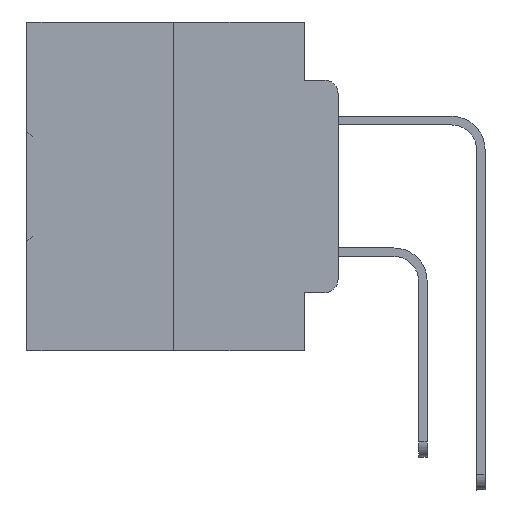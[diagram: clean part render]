
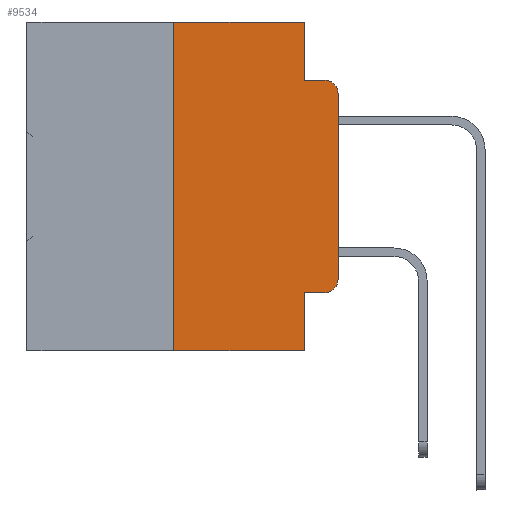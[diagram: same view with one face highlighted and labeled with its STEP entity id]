
A CAD part, left-side view. The second image highlights one B-rep face of the part: STEP entity #9534.
In plain terms, the highlighted planar face has unit normal (-1, 0, 0).
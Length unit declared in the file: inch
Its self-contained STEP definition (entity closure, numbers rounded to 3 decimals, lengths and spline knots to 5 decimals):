
#458 = CARTESIAN_POINT ( 'NONE',  ( 0., 0.25, -0.5 ) ) ;
#621 = ORIENTED_EDGE ( 'NONE', *, *, #17937, .F. ) ;
#1419 = VECTOR ( 'NONE', #21801, 39.37008 ) ;
#1692 = AXIS2_PLACEMENT_3D ( 'NONE', #29092, #12473, #31791 ) ;
#1959 = EDGE_CURVE ( 'NONE', #13216, #26898, #23651, .T. ) ;
#2672 = DIRECTION ( 'NONE',  ( 0., 0., -1. ) ) ;
#3133 = CARTESIAN_POINT ( 'NONE',  ( 0., 0.473, 0. ) ) ;
#4731 = DIRECTION ( 'NONE',  ( 0., -1., 0. ) ) ;
#5569 = ORIENTED_EDGE ( 'NONE', *, *, #9175, .T. ) ;
#5949 = CARTESIAN_POINT ( 'NONE',  ( 0., 0.02, -0.3915 ) ) ;
#6005 = DIRECTION ( 'NONE',  ( 0., -1., 0. ) ) ;
#6190 = ORIENTED_EDGE ( 'NONE', *, *, #30833, .T. ) ;
#6446 = CARTESIAN_POINT ( 'NONE',  ( 0., 0.473, -0.5 ) ) ;
#6785 = CARTESIAN_POINT ( 'NONE',  ( 0., 0.051, -0.4115 ) ) ;
#7320 = LINE ( 'NONE', #27417, #8239 ) ;
#7840 = VECTOR ( 'NONE', #34298, 39.37008 ) ;
#8078 = AXIS2_PLACEMENT_3D ( 'NONE', #5949, #25584, #8837 ) ;
#8204 = LINE ( 'NONE', #13092, #22275 ) ;
#8239 = VECTOR ( 'NONE', #10777, 39.37008 ) ;
#8837 = DIRECTION ( 'NONE',  ( 0., 0., -1. ) ) ;
#8982 = CARTESIAN_POINT ( 'NONE',  ( 0., 0., -0.3915 ) ) ;
#9175 = EDGE_CURVE ( 'NONE', #9709, #26898, #31690, .T. ) ;
#9199 = CARTESIAN_POINT ( 'NONE',  ( 0., 0., -0.1085 ) ) ;
#9534 = ADVANCED_FACE ( 'NONE', ( #34170 ), #14041, .F. ) ;
#9709 = VERTEX_POINT ( 'NONE', #9199 ) ;
#9839 = ORIENTED_EDGE ( 'NONE', *, *, #16330, .F. ) ;
#10165 = CARTESIAN_POINT ( 'NONE',  ( 0., 0.051, -0.5 ) ) ;
#10264 = VERTEX_POINT ( 'NONE', #27933 ) ;
#10777 = DIRECTION ( 'NONE',  ( 0., 0., -1. ) ) ;
#10989 = ORIENTED_EDGE ( 'NONE', *, *, #12405, .T. ) ;
#11061 = LINE ( 'NONE', #3133, #25013 ) ;
#11321 = ORIENTED_EDGE ( 'NONE', *, *, #28328, .T. ) ;
#11928 = DIRECTION ( 'NONE',  ( 0., 0., 1. ) ) ;
#12405 = EDGE_CURVE ( 'NONE', #23064, #19963, #16854, .T. ) ;
#12473 = DIRECTION ( 'NONE',  ( -1., 0., 0. ) ) ;
#13092 = CARTESIAN_POINT ( 'NONE',  ( 0., 0.051, -0.4115 ) ) ;
#13216 = VERTEX_POINT ( 'NONE', #16215 ) ;
#13557 = DIRECTION ( 'NONE',  ( 0., 0., 1. ) ) ;
#14041 = PLANE ( 'NONE',  #18158 ) ;
#14109 = EDGE_CURVE ( 'NONE', #23976, #33843, #28851, .T. ) ;
#15780 = CARTESIAN_POINT ( 'NONE',  ( 0., 0.02, -0.0885 ) ) ;
#16215 = CARTESIAN_POINT ( 'NONE',  ( 0., 0.051, -0.0885 ) ) ;
#16330 = EDGE_CURVE ( 'NONE', #32833, #19963, #31224, .T. ) ;
#16854 = LINE ( 'NONE', #6446, #31445 ) ;
#17543 = CARTESIAN_POINT ( 'NONE',  ( 0., 0.02, -0.4115 ) ) ;
#17937 = EDGE_CURVE ( 'NONE', #23064, #25460, #31519, .T. ) ;
#18158 = AXIS2_PLACEMENT_3D ( 'NONE', #35959, #19687, #2672 ) ;
#18593 = ORIENTED_EDGE ( 'NONE', *, *, #30388, .F. ) ;
#19687 = DIRECTION ( 'NONE',  ( 1., 0., 0. ) ) ;
#19963 = VERTEX_POINT ( 'NONE', #10165 ) ;
#21668 = ORIENTED_EDGE ( 'NONE', *, *, #1959, .F. ) ;
#21801 = DIRECTION ( 'NONE',  ( 0., 0., -1. ) ) ;
#22275 = VECTOR ( 'NONE', #4731, 39.37008 ) ;
#23064 = VERTEX_POINT ( 'NONE', #458 ) ;
#23651 = LINE ( 'NONE', #33423, #7840 ) ;
#23976 = VERTEX_POINT ( 'NONE', #17543 ) ;
#24268 = VECTOR ( 'NONE', #11928, 39.37008 ) ;
#24326 = CARTESIAN_POINT ( 'NONE',  ( 0., 0.25, 0. ) ) ;
#24587 = CARTESIAN_POINT ( 'NONE',  ( 0., 0.051, 0. ) ) ;
#24621 = ORIENTED_EDGE ( 'NONE', *, *, #14109, .T. ) ;
#25013 = VECTOR ( 'NONE', #6005, 39.37008 ) ;
#25111 = VECTOR ( 'NONE', #13557, 39.37008 ) ;
#25460 = VERTEX_POINT ( 'NONE', #24326 ) ;
#25584 = DIRECTION ( 'NONE',  ( -1., 0., 0. ) ) ;
#26051 = DIRECTION ( 'NONE',  ( 0., -1., 0. ) ) ;
#26112 = EDGE_LOOP ( 'NONE', ( #11321, #5569, #21668, #18593, #33271, #621, #10989, #9839, #6190, #24621 ) ) ;
#26898 = VERTEX_POINT ( 'NONE', #15780 ) ;
#27260 = CARTESIAN_POINT ( 'NONE',  ( 0., 0., 0. ) ) ;
#27417 = CARTESIAN_POINT ( 'NONE',  ( 0., 0.051, 0. ) ) ;
#27933 = CARTESIAN_POINT ( 'NONE',  ( 0., 0.051, 0. ) ) ;
#28328 = EDGE_CURVE ( 'NONE', #33843, #9709, #32337, .T. ) ;
#28851 = CIRCLE ( 'NONE', #8078, 0.02 ) ;
#29092 = CARTESIAN_POINT ( 'NONE',  ( 0., 0.02, -0.1085 ) ) ;
#30388 = EDGE_CURVE ( 'NONE', #10264, #13216, #7320, .T. ) ;
#30833 = EDGE_CURVE ( 'NONE', #32833, #23976, #8204, .T. ) ;
#31224 = LINE ( 'NONE', #24587, #1419 ) ;
#31270 = CARTESIAN_POINT ( 'NONE',  ( 0., 0.25, 0. ) ) ;
#31445 = VECTOR ( 'NONE', #26051, 39.37008 ) ;
#31519 = LINE ( 'NONE', #31270, #24268 ) ;
#31690 = CIRCLE ( 'NONE', #1692, 0.02 ) ;
#31791 = DIRECTION ( 'NONE',  ( 0., 0., -1. ) ) ;
#32337 = LINE ( 'NONE', #27260, #25111 ) ;
#32833 = VERTEX_POINT ( 'NONE', #6785 ) ;
#33271 = ORIENTED_EDGE ( 'NONE', *, *, #35067, .F. ) ;
#33423 = CARTESIAN_POINT ( 'NONE',  ( 0., 0.051, -0.0885 ) ) ;
#33843 = VERTEX_POINT ( 'NONE', #8982 ) ;
#34170 = FACE_OUTER_BOUND ( 'NONE', #26112, .T. ) ;
#34298 = DIRECTION ( 'NONE',  ( 0., -1., 0. ) ) ;
#35067 = EDGE_CURVE ( 'NONE', #25460, #10264, #11061, .T. ) ;
#35959 = CARTESIAN_POINT ( 'NONE',  ( 0., 0.473, 0. ) ) ;
